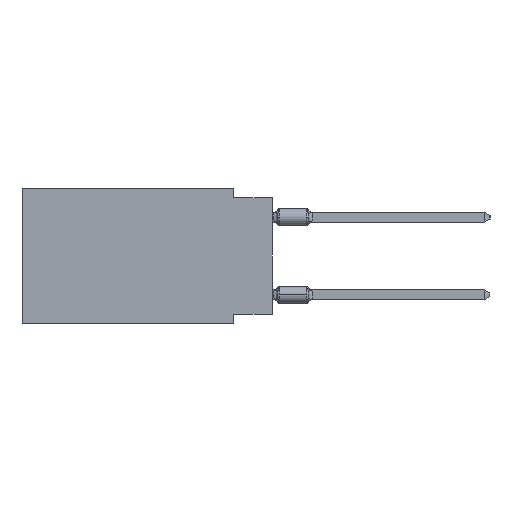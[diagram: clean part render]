
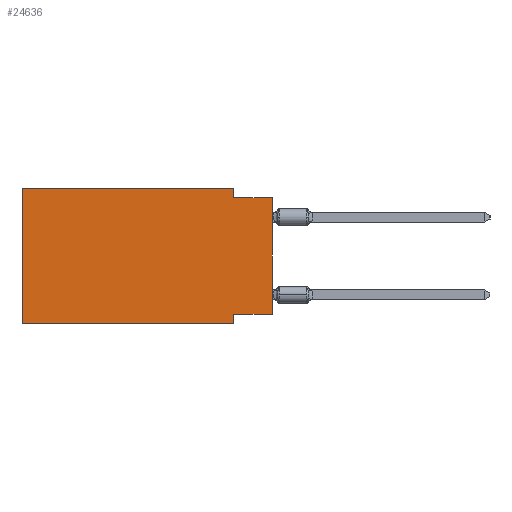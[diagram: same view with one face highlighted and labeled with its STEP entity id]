
A CAD part, left-side view. The second image highlights one B-rep face of the part: STEP entity #24636.
In plain terms, the highlighted planar face has unit normal (-1, 0, 0).
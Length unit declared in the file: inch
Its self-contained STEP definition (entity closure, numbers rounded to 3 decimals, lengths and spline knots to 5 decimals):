
#1080 = VERTEX_POINT ( 'NONE', #20681 ) ;
#1189 = EDGE_CURVE ( 'NONE', #1080, #2051, #31516, .T. ) ;
#1397 = CARTESIAN_POINT ( 'NONE',  ( 0., 0., -0.025 ) ) ;
#1847 = PLANE ( 'NONE',  #34761 ) ;
#1889 = DIRECTION ( 'NONE',  ( 0., 0., -1. ) ) ;
#2051 = VERTEX_POINT ( 'NONE', #6032 ) ;
#2090 = CARTESIAN_POINT ( 'NONE',  ( 0., 0.1, -0.325 ) ) ;
#3335 = VECTOR ( 'NONE', #1889, 39.37008 ) ;
#3344 = ORIENTED_EDGE ( 'NONE', *, *, #14547, .F. ) ;
#4205 = CARTESIAN_POINT ( 'NONE',  ( 0., 0.645, 0. ) ) ;
#4861 = EDGE_CURVE ( 'NONE', #7573, #15689, #16585, .T. ) ;
#6032 = CARTESIAN_POINT ( 'NONE',  ( 0., 0.1, -0.35 ) ) ;
#7573 = VERTEX_POINT ( 'NONE', #21788 ) ;
#7706 = ORIENTED_EDGE ( 'NONE', *, *, #4861, .F. ) ;
#8439 = CARTESIAN_POINT ( 'NONE',  ( 0., 0.1, 0. ) ) ;
#8657 = CARTESIAN_POINT ( 'NONE',  ( 0., 0., 0. ) ) ;
#9039 = CARTESIAN_POINT ( 'NONE',  ( 0., 0., -0.325 ) ) ;
#9373 = CARTESIAN_POINT ( 'NONE',  ( 0., 0., -0.025 ) ) ;
#14547 = EDGE_CURVE ( 'NONE', #25061, #7573, #34402, .T. ) ;
#14783 = VECTOR ( 'NONE', #19489, 39.37008 ) ;
#15248 = EDGE_CURVE ( 'NONE', #33435, #33153, #30737, .T. ) ;
#15602 = DIRECTION ( 'NONE',  ( 1., 0., 0. ) ) ;
#15689 = VERTEX_POINT ( 'NONE', #25648 ) ;
#15947 = FACE_OUTER_BOUND ( 'NONE', #17516, .T. ) ;
#16141 = VECTOR ( 'NONE', #25730, 39.37008 ) ;
#16585 = LINE ( 'NONE', #8439, #14783 ) ;
#17516 = EDGE_LOOP ( 'NONE', ( #23664, #30418, #7706, #3344, #30909, #27428, #22624, #33532 ) ) ;
#18122 = LINE ( 'NONE', #26606, #19180 ) ;
#18134 = DIRECTION ( 'NONE',  ( 0., -1., 0. ) ) ;
#19180 = VECTOR ( 'NONE', #34754, 39.37008 ) ;
#19337 = DIRECTION ( 'NONE',  ( 0., 0., 1. ) ) ;
#19489 = DIRECTION ( 'NONE',  ( 0., 0., -1. ) ) ;
#20500 = CARTESIAN_POINT ( 'NONE',  ( 0., 0.645, -0.35 ) ) ;
#20681 = CARTESIAN_POINT ( 'NONE',  ( 0., 0.645, -0.35 ) ) ;
#21788 = CARTESIAN_POINT ( 'NONE',  ( 0., 0.1, 0. ) ) ;
#22507 = EDGE_CURVE ( 'NONE', #33435, #22947, #18122, .T. ) ;
#22624 = ORIENTED_EDGE ( 'NONE', *, *, #28268, .F. ) ;
#22855 = EDGE_CURVE ( 'NONE', #15689, #33153, #26174, .T. ) ;
#22947 = VERTEX_POINT ( 'NONE', #2090 ) ;
#23471 = DIRECTION ( 'NONE',  ( 0., -1., 0. ) ) ;
#23664 = ORIENTED_EDGE ( 'NONE', *, *, #15248, .T. ) ;
#24636 = ADVANCED_FACE ( 'NONE', ( #15947 ), #1847, .F. ) ;
#24673 = VECTOR ( 'NONE', #19337, 39.37008 ) ;
#24953 = VECTOR ( 'NONE', #34494, 39.37008 ) ;
#24956 = VECTOR ( 'NONE', #23471, 39.37008 ) ;
#25061 = VERTEX_POINT ( 'NONE', #27115 ) ;
#25648 = CARTESIAN_POINT ( 'NONE',  ( 0., 0.1, -0.025 ) ) ;
#25730 = DIRECTION ( 'NONE',  ( 0., -1., 0. ) ) ;
#26174 = LINE ( 'NONE', #1397, #24956 ) ;
#26491 = LINE ( 'NONE', #35342, #3335 ) ;
#26606 = CARTESIAN_POINT ( 'NONE',  ( 0., 0., -0.325 ) ) ;
#26970 = CARTESIAN_POINT ( 'NONE',  ( 0., 0.645, 0. ) ) ;
#27115 = CARTESIAN_POINT ( 'NONE',  ( 0., 0.645, 0. ) ) ;
#27428 = ORIENTED_EDGE ( 'NONE', *, *, #1189, .T. ) ;
#28268 = EDGE_CURVE ( 'NONE', #22947, #2051, #26491, .T. ) ;
#28922 = LINE ( 'NONE', #32120, #24953 ) ;
#29282 = VECTOR ( 'NONE', #18134, 39.37008 ) ;
#30418 = ORIENTED_EDGE ( 'NONE', *, *, #22855, .F. ) ;
#30737 = LINE ( 'NONE', #8657, #24673 ) ;
#30909 = ORIENTED_EDGE ( 'NONE', *, *, #33141, .F. ) ;
#31516 = LINE ( 'NONE', #20500, #16141 ) ;
#32120 = CARTESIAN_POINT ( 'NONE',  ( 0., 0.645, 0. ) ) ;
#33141 = EDGE_CURVE ( 'NONE', #1080, #25061, #28922, .T. ) ;
#33153 = VERTEX_POINT ( 'NONE', #9373 ) ;
#33435 = VERTEX_POINT ( 'NONE', #9039 ) ;
#33532 = ORIENTED_EDGE ( 'NONE', *, *, #22507, .F. ) ;
#34402 = LINE ( 'NONE', #4205, #29282 ) ;
#34494 = DIRECTION ( 'NONE',  ( 0., 0., 1. ) ) ;
#34754 = DIRECTION ( 'NONE',  ( 0., 1., 0. ) ) ;
#34761 = AXIS2_PLACEMENT_3D ( 'NONE', #26970, #15602, #35469 ) ;
#35342 = CARTESIAN_POINT ( 'NONE',  ( 0., 0.1, -0.35 ) ) ;
#35469 = DIRECTION ( 'NONE',  ( 0., 0., -1. ) ) ;
